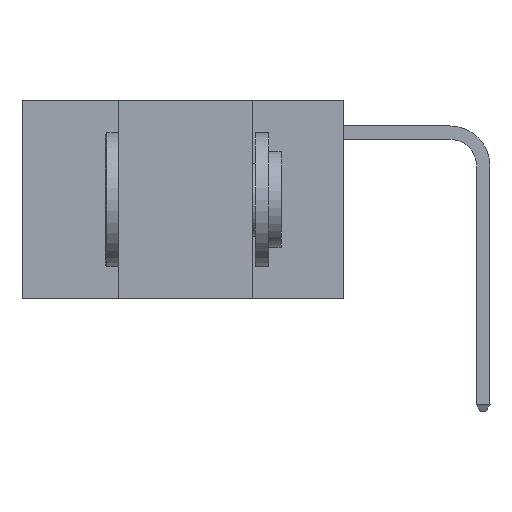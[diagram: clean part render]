
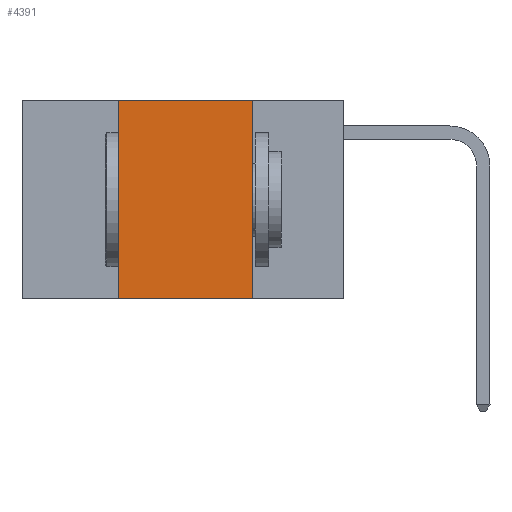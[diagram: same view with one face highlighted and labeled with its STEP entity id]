
A CAD part, left-side view. The second image highlights one B-rep face of the part: STEP entity #4391.
In plain terms, the highlighted planar face has unit normal (-1, 0, 0).
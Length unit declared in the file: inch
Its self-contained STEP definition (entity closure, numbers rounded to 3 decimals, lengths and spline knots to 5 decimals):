
#400 = FACE_OUTER_BOUND ( 'NONE', #6157, .T. ) ;
#414 = DIRECTION ( 'NONE',  ( 0., -1., 0. ) ) ;
#1797 = CARTESIAN_POINT ( 'NONE',  ( 0., 0.6, 0. ) ) ;
#1830 = DIRECTION ( 'NONE',  ( 0., -1., 0. ) ) ;
#2010 = ORIENTED_EDGE ( 'NONE', *, *, #12134, .F. ) ;
#3356 = VECTOR ( 'NONE', #15499, 39.37008 ) ;
#3579 = DIRECTION ( 'NONE',  ( 0., 0., -1. ) ) ;
#4391 = ADVANCED_FACE ( 'NONE', ( #400 ), #5039, .F. ) ;
#4852 = CARTESIAN_POINT ( 'NONE',  ( 0., 0.42, 0. ) ) ;
#4887 = LINE ( 'NONE', #14204, #18865 ) ;
#5039 = PLANE ( 'NONE',  #13030 ) ;
#6157 = EDGE_LOOP ( 'NONE', ( #16358, #2010, #12636, #12229 ) ) ;
#6231 = VERTEX_POINT ( 'NONE', #18921 ) ;
#7869 = LINE ( 'NONE', #14005, #3356 ) ;
#9804 = VERTEX_POINT ( 'NONE', #19450 ) ;
#10659 = CARTESIAN_POINT ( 'NONE',  ( 0., 0.42, 0. ) ) ;
#10693 = DIRECTION ( 'NONE',  ( 1., 0., 0. ) ) ;
#11761 = VERTEX_POINT ( 'NONE', #4852 ) ;
#12134 = EDGE_CURVE ( 'NONE', #11761, #9804, #4887, .T. ) ;
#12206 = EDGE_CURVE ( 'NONE', #9804, #6231, #7869, .T. ) ;
#12229 = ORIENTED_EDGE ( 'NONE', *, *, #17902, .T. ) ;
#12636 = ORIENTED_EDGE ( 'NONE', *, *, #18652, .F. ) ;
#13030 = AXIS2_PLACEMENT_3D ( 'NONE', #1797, #10693, #3579 ) ;
#14005 = CARTESIAN_POINT ( 'NONE',  ( 0., 0.17, 0. ) ) ;
#14186 = LINE ( 'NONE', #17355, #16183 ) ;
#14204 = CARTESIAN_POINT ( 'NONE',  ( 0., 0.6, 0. ) ) ;
#15458 = CARTESIAN_POINT ( 'NONE',  ( 0., 0.42, -0.37 ) ) ;
#15499 = DIRECTION ( 'NONE',  ( 0., 0., -1. ) ) ;
#16183 = VECTOR ( 'NONE', #414, 39.37008 ) ;
#16358 = ORIENTED_EDGE ( 'NONE', *, *, #12206, .F. ) ;
#16479 = VECTOR ( 'NONE', #16731, 39.37008 ) ;
#16731 = DIRECTION ( 'NONE',  ( 0., 0., 1. ) ) ;
#17355 = CARTESIAN_POINT ( 'NONE',  ( 0., 0.6, -0.37 ) ) ;
#17902 = EDGE_CURVE ( 'NONE', #18272, #6231, #14186, .T. ) ;
#18217 = LINE ( 'NONE', #10659, #16479 ) ;
#18272 = VERTEX_POINT ( 'NONE', #15458 ) ;
#18652 = EDGE_CURVE ( 'NONE', #18272, #11761, #18217, .T. ) ;
#18865 = VECTOR ( 'NONE', #1830, 39.37008 ) ;
#18921 = CARTESIAN_POINT ( 'NONE',  ( 0., 0.17, -0.37 ) ) ;
#19450 = CARTESIAN_POINT ( 'NONE',  ( 0., 0.17, 0. ) ) ;
